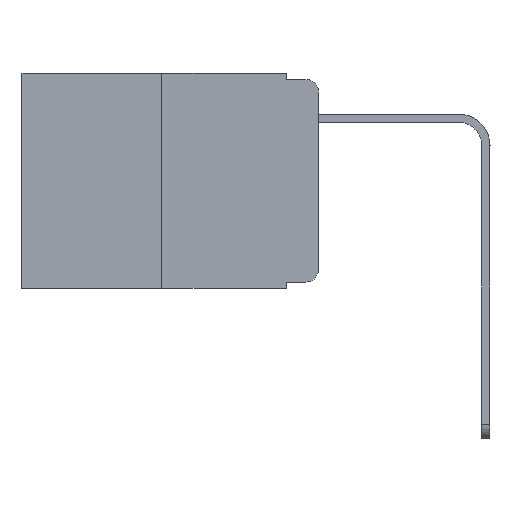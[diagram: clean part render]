
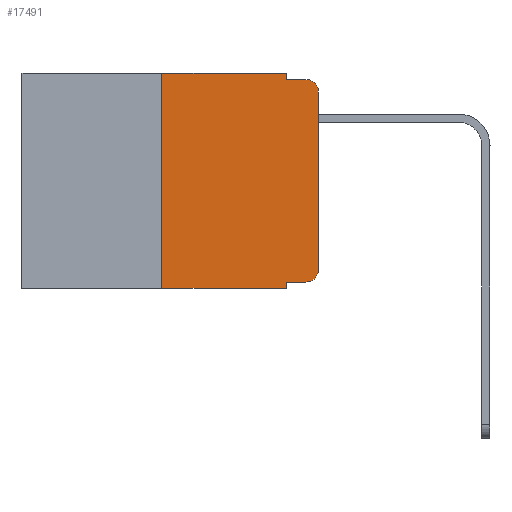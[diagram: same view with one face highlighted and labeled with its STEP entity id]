
A CAD part, left-side view. The second image highlights one B-rep face of the part: STEP entity #17491.
In plain terms, the highlighted planar face has unit normal (-1, 0, 0).
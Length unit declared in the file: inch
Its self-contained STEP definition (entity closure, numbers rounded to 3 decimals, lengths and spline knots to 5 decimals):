
#28 = VERTEX_POINT ( 'NONE', #16398 ) ;
#142 = CARTESIAN_POINT ( 'NONE',  ( 0., 0.051, -0.01 ) ) ;
#181 = VECTOR ( 'NONE', #16672, 39.37008 ) ;
#275 = VECTOR ( 'NONE', #7073, 39.37008 ) ;
#431 = CARTESIAN_POINT ( 'NONE',  ( 0., 0.02, -0.333 ) ) ;
#480 = ORIENTED_EDGE ( 'NONE', *, *, #16283, .F. ) ;
#536 = LINE ( 'NONE', #19467, #275 ) ;
#647 = ORIENTED_EDGE ( 'NONE', *, *, #8432, .F. ) ;
#686 = VECTOR ( 'NONE', #8651, 39.37008 ) ;
#1060 = DIRECTION ( 'NONE',  ( -1., 0., 0. ) ) ;
#1706 = VERTEX_POINT ( 'NONE', #14354 ) ;
#1787 = LINE ( 'NONE', #16486, #14870 ) ;
#2190 = LINE ( 'NONE', #13102, #16732 ) ;
#2425 = ORIENTED_EDGE ( 'NONE', *, *, #4541, .T. ) ;
#2739 = ORIENTED_EDGE ( 'NONE', *, *, #17020, .F. ) ;
#3127 = ORIENTED_EDGE ( 'NONE', *, *, #15453, .F. ) ;
#3651 = VERTEX_POINT ( 'NONE', #8078 ) ;
#4017 = ORIENTED_EDGE ( 'NONE', *, *, #11981, .T. ) ;
#4092 = FACE_OUTER_BOUND ( 'NONE', #11100, .T. ) ;
#4187 = CARTESIAN_POINT ( 'NONE',  ( 0., 0.02, -0.313 ) ) ;
#4419 = CARTESIAN_POINT ( 'NONE',  ( 0., 0.02, -0.03 ) ) ;
#4541 = EDGE_CURVE ( 'NONE', #11231, #15462, #16605, .T. ) ;
#4547 = CARTESIAN_POINT ( 'NONE',  ( 0., 0.051, 0. ) ) ;
#4762 = VERTEX_POINT ( 'NONE', #142 ) ;
#5085 = EDGE_CURVE ( 'NONE', #8132, #3651, #536, .T. ) ;
#5436 = VECTOR ( 'NONE', #5841, 39.37008 ) ;
#5841 = DIRECTION ( 'NONE',  ( 0., 0., 1. ) ) ;
#6084 = ORIENTED_EDGE ( 'NONE', *, *, #5085, .F. ) ;
#6161 = EDGE_CURVE ( 'NONE', #15462, #28, #20218, .T. ) ;
#7073 = DIRECTION ( 'NONE',  ( 0., 0., -1. ) ) ;
#7074 = DIRECTION ( 'NONE',  ( 0., -1., 0. ) ) ;
#7409 = ORIENTED_EDGE ( 'NONE', *, *, #6161, .T. ) ;
#7646 = DIRECTION ( 'NONE',  ( 0., 0., -1. ) ) ;
#8078 = CARTESIAN_POINT ( 'NONE',  ( 0., 0.051, -0.343 ) ) ;
#8132 = VERTEX_POINT ( 'NONE', #9550 ) ;
#8233 = ORIENTED_EDGE ( 'NONE', *, *, #12193, .T. ) ;
#8432 = EDGE_CURVE ( 'NONE', #15222, #16006, #20410, .T. ) ;
#8610 = DIRECTION ( 'NONE',  ( 0., -1., 0. ) ) ;
#8651 = DIRECTION ( 'NONE',  ( 0., 0., 1. ) ) ;
#9157 = CARTESIAN_POINT ( 'NONE',  ( 0., 0., 0. ) ) ;
#9208 = DIRECTION ( 'NONE',  ( 1., 0., 0. ) ) ;
#9550 = CARTESIAN_POINT ( 'NONE',  ( 0., 0.051, -0.333 ) ) ;
#9754 = ORIENTED_EDGE ( 'NONE', *, *, #9855, .T. ) ;
#9855 = EDGE_CURVE ( 'NONE', #28, #19747, #10275, .T. ) ;
#10275 = CIRCLE ( 'NONE', #13145, 0.02 ) ;
#10337 = CARTESIAN_POINT ( 'NONE',  ( 0., 0.473, 0. ) ) ;
#11100 = EDGE_LOOP ( 'NONE', ( #7409, #9754, #3127, #2739, #480, #647, #8233, #6084, #4017, #2425 ) ) ;
#11147 = CARTESIAN_POINT ( 'NONE',  ( 0., 0.25, -0.343 ) ) ;
#11231 = VERTEX_POINT ( 'NONE', #431 ) ;
#11279 = CARTESIAN_POINT ( 'NONE',  ( 0., 0.25, 0. ) ) ;
#11981 = EDGE_CURVE ( 'NONE', #8132, #11231, #1787, .T. ) ;
#12088 = DIRECTION ( 'NONE',  ( 0., 0., -1. ) ) ;
#12193 = EDGE_CURVE ( 'NONE', #15222, #3651, #19295, .T. ) ;
#12683 = LINE ( 'NONE', #4547, #16383 ) ;
#13069 = CARTESIAN_POINT ( 'NONE',  ( 0., 0.473, -0.343 ) ) ;
#13102 = CARTESIAN_POINT ( 'NONE',  ( 0., 0.051, -0.01 ) ) ;
#13145 = AXIS2_PLACEMENT_3D ( 'NONE', #4419, #17008, #12088 ) ;
#13185 = CARTESIAN_POINT ( 'NONE',  ( 0., 0., -0.313 ) ) ;
#13214 = AXIS2_PLACEMENT_3D ( 'NONE', #4187, #1060, #15193 ) ;
#13221 = CARTESIAN_POINT ( 'NONE',  ( 0., 0.02, -0.01 ) ) ;
#13554 = PLANE ( 'NONE',  #16505 ) ;
#14354 = CARTESIAN_POINT ( 'NONE',  ( 0., 0.051, 0. ) ) ;
#14742 = DIRECTION ( 'NONE',  ( 0., -1., 0. ) ) ;
#14870 = VECTOR ( 'NONE', #7074, 39.37008 ) ;
#15193 = DIRECTION ( 'NONE',  ( 0., 0., -1. ) ) ;
#15222 = VERTEX_POINT ( 'NONE', #11147 ) ;
#15453 = EDGE_CURVE ( 'NONE', #4762, #19747, #2190, .T. ) ;
#15462 = VERTEX_POINT ( 'NONE', #13185 ) ;
#16006 = VERTEX_POINT ( 'NONE', #11279 ) ;
#16283 = EDGE_CURVE ( 'NONE', #16006, #1706, #19165, .T. ) ;
#16383 = VECTOR ( 'NONE', #17274, 39.37008 ) ;
#16398 = CARTESIAN_POINT ( 'NONE',  ( 0., 0., -0.03 ) ) ;
#16486 = CARTESIAN_POINT ( 'NONE',  ( 0., 0.051, -0.333 ) ) ;
#16505 = AXIS2_PLACEMENT_3D ( 'NONE', #16703, #9208, #7646 ) ;
#16605 = CIRCLE ( 'NONE', #13214, 0.02 ) ;
#16672 = DIRECTION ( 'NONE',  ( 0., -1., 0. ) ) ;
#16703 = CARTESIAN_POINT ( 'NONE',  ( 0., 0.473, 0. ) ) ;
#16732 = VECTOR ( 'NONE', #14742, 39.37008 ) ;
#17008 = DIRECTION ( 'NONE',  ( -1., 0., 0. ) ) ;
#17020 = EDGE_CURVE ( 'NONE', #1706, #4762, #12683, .T. ) ;
#17274 = DIRECTION ( 'NONE',  ( 0., 0., -1. ) ) ;
#17491 = ADVANCED_FACE ( 'NONE', ( #4092 ), #13554, .F. ) ;
#18006 = CARTESIAN_POINT ( 'NONE',  ( 0., 0.25, 0. ) ) ;
#18296 = VECTOR ( 'NONE', #8610, 39.37008 ) ;
#19165 = LINE ( 'NONE', #10337, #181 ) ;
#19295 = LINE ( 'NONE', #13069, #18296 ) ;
#19467 = CARTESIAN_POINT ( 'NONE',  ( 0., 0.051, 0. ) ) ;
#19747 = VERTEX_POINT ( 'NONE', #13221 ) ;
#20218 = LINE ( 'NONE', #9157, #5436 ) ;
#20410 = LINE ( 'NONE', #18006, #686 ) ;
